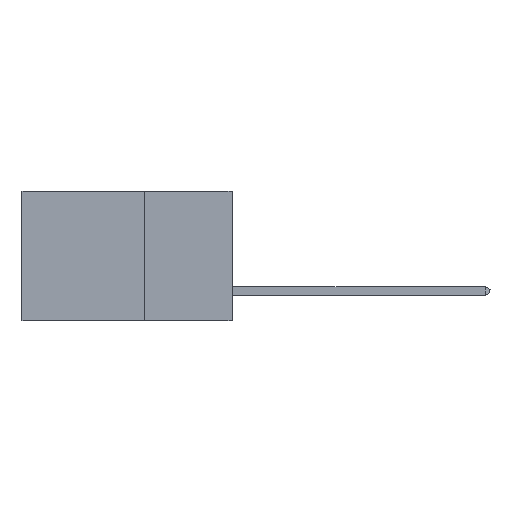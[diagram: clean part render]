
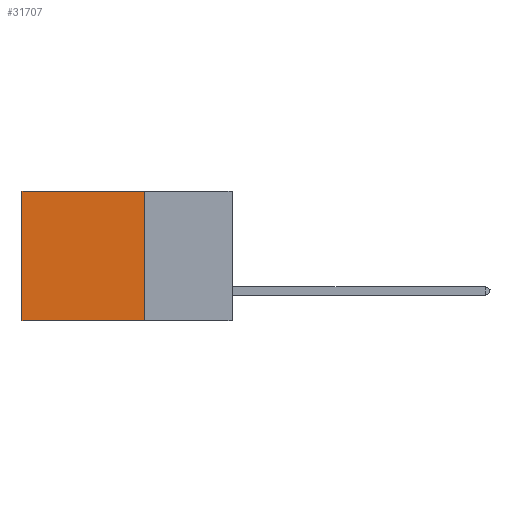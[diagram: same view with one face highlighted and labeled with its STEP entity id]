
A CAD part, left-side view. The second image highlights one B-rep face of the part: STEP entity #31707.
In plain terms, the highlighted planar face has unit normal (-1, 0, 0).
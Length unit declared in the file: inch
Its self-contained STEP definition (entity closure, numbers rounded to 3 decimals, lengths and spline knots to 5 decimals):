
#340 = LINE ( 'NONE', #23815, #25509 ) ;
#731 = DIRECTION ( 'NONE',  ( 0., 1., 0. ) ) ;
#3298 = ORIENTED_EDGE ( 'NONE', *, *, #35509, .F. ) ;
#3352 = CARTESIAN_POINT ( 'NONE',  ( 0.2875, 0.25, 0. ) ) ;
#5621 = LINE ( 'NONE', #16737, #27370 ) ;
#6274 = DIRECTION ( 'NONE',  ( 1., 0., 0. ) ) ;
#9449 = VERTEX_POINT ( 'NONE', #19027 ) ;
#9892 = ORIENTED_EDGE ( 'NONE', *, *, #31273, .T. ) ;
#11697 = DIRECTION ( 'NONE',  ( 0., 1., 0. ) ) ;
#13155 = VECTOR ( 'NONE', #11697, 39.37008 ) ;
#14565 = CARTESIAN_POINT ( 'NONE',  ( 0.2875, 0.6, 0. ) ) ;
#16253 = EDGE_CURVE ( 'NONE', #33207, #26160, #39811, .T. ) ;
#16737 = CARTESIAN_POINT ( 'NONE',  ( 0.2875, 0.25, 0. ) ) ;
#18263 = ORIENTED_EDGE ( 'NONE', *, *, #34468, .T. ) ;
#19027 = CARTESIAN_POINT ( 'NONE',  ( 0.2875, 0.25, 0. ) ) ;
#23098 = LINE ( 'NONE', #3352, #24510 ) ;
#23815 = CARTESIAN_POINT ( 'NONE',  ( 0.2875, 0.6, 0. ) ) ;
#23928 = CARTESIAN_POINT ( 'NONE',  ( 0.2875, 0.25, -0.37 ) ) ;
#24510 = VECTOR ( 'NONE', #731, 39.37008 ) ;
#25509 = VECTOR ( 'NONE', #38988, 39.37008 ) ;
#26160 = VERTEX_POINT ( 'NONE', #29434 ) ;
#27370 = VECTOR ( 'NONE', #31338, 39.37008 ) ;
#27905 = CARTESIAN_POINT ( 'NONE',  ( 0.2875, 0.25, 0. ) ) ;
#28035 = DIRECTION ( 'NONE',  ( 0., 0., -1. ) ) ;
#29434 = CARTESIAN_POINT ( 'NONE',  ( 0.2875, 0.6, -0.37 ) ) ;
#29753 = EDGE_LOOP ( 'NONE', ( #18263, #39252, #3298, #9892 ) ) ;
#30320 = FACE_OUTER_BOUND ( 'NONE', #29753, .T. ) ;
#31145 = PLANE ( 'NONE',  #34720 ) ;
#31273 = EDGE_CURVE ( 'NONE', #9449, #37975, #23098, .T. ) ;
#31338 = DIRECTION ( 'NONE',  ( 0., 0., -1. ) ) ;
#31707 = ADVANCED_FACE ( 'NONE', ( #30320 ), #31145, .F. ) ;
#33207 = VERTEX_POINT ( 'NONE', #23928 ) ;
#34468 = EDGE_CURVE ( 'NONE', #37975, #26160, #340, .T. ) ;
#34720 = AXIS2_PLACEMENT_3D ( 'NONE', #27905, #6274, #28035 ) ;
#35509 = EDGE_CURVE ( 'NONE', #9449, #33207, #5621, .T. ) ;
#36117 = CARTESIAN_POINT ( 'NONE',  ( 0.2875, 0.25, -0.37 ) ) ;
#37975 = VERTEX_POINT ( 'NONE', #14565 ) ;
#38988 = DIRECTION ( 'NONE',  ( 0., 0., -1. ) ) ;
#39252 = ORIENTED_EDGE ( 'NONE', *, *, #16253, .F. ) ;
#39811 = LINE ( 'NONE', #36117, #13155 ) ;
